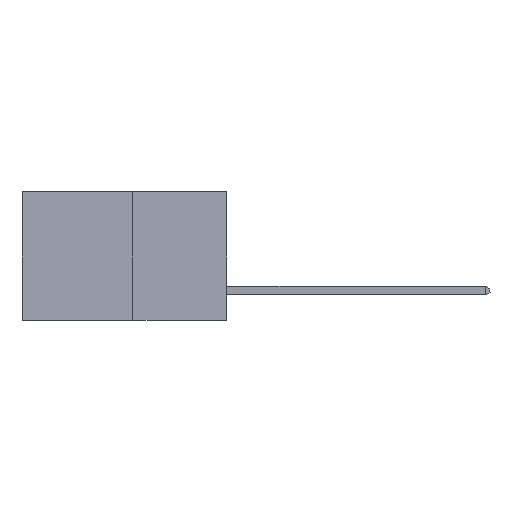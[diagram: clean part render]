
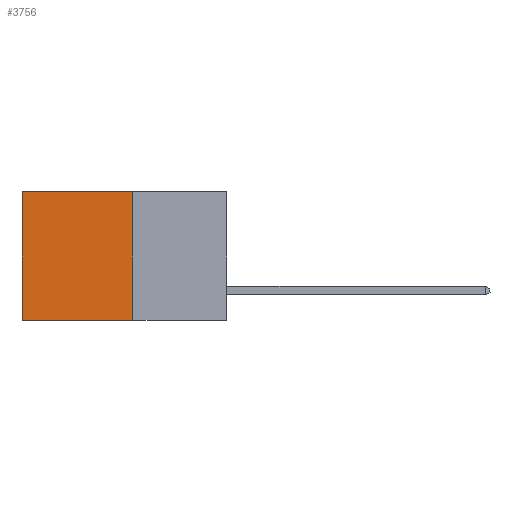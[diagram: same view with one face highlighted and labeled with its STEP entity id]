
A CAD part, left-side view. The second image highlights one B-rep face of the part: STEP entity #3756.
In plain terms, the highlighted planar face has unit normal (-1, 0, 0).
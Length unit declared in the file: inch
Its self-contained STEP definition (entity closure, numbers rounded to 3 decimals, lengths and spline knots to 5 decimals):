
#279 = VECTOR ( 'NONE', #6995, 39.37008 ) ;
#903 = VECTOR ( 'NONE', #10821, 39.37008 ) ;
#1159 = EDGE_LOOP ( 'NONE', ( #3875, #5077, #8841, #7948 ) ) ;
#1236 = VERTEX_POINT ( 'NONE', #6730 ) ;
#1949 = DIRECTION ( 'NONE',  ( 0., 0., -1. ) ) ;
#2069 = CARTESIAN_POINT ( 'NONE',  ( 0.277, 0.27, -0.37 ) ) ;
#2917 = VERTEX_POINT ( 'NONE', #6282 ) ;
#2950 = VECTOR ( 'NONE', #1949, 39.37008 ) ;
#3147 = VECTOR ( 'NONE', #10417, 39.37008 ) ;
#3756 = ADVANCED_FACE ( 'NONE', ( #9058 ), #8468, .F. ) ;
#3875 = ORIENTED_EDGE ( 'NONE', *, *, #9481, .T. ) ;
#3939 = EDGE_CURVE ( 'NONE', #10546, #2917, #5528, .T. ) ;
#4359 = AXIS2_PLACEMENT_3D ( 'NONE', #8403, #8313, #8305 ) ;
#4400 = EDGE_CURVE ( 'NONE', #1236, #10546, #7510, .T. ) ;
#4759 = VERTEX_POINT ( 'NONE', #7749 ) ;
#5077 = ORIENTED_EDGE ( 'NONE', *, *, #3939, .F. ) ;
#5528 = LINE ( 'NONE', #6834, #279 ) ;
#6083 = LINE ( 'NONE', #10022, #903 ) ;
#6282 = CARTESIAN_POINT ( 'NONE',  ( 0.277, 0.59, -0.37 ) ) ;
#6730 = CARTESIAN_POINT ( 'NONE',  ( 0.277, 0.27, 0. ) ) ;
#6834 = CARTESIAN_POINT ( 'NONE',  ( 0.277, 0.27, -0.37 ) ) ;
#6995 = DIRECTION ( 'NONE',  ( 0., 1., 0. ) ) ;
#7244 = CARTESIAN_POINT ( 'NONE',  ( 0.277, 0.27, 0. ) ) ;
#7380 = EDGE_CURVE ( 'NONE', #1236, #4759, #9361, .T. ) ;
#7510 = LINE ( 'NONE', #2069, #2950 ) ;
#7749 = CARTESIAN_POINT ( 'NONE',  ( 0.277, 0.59, 0. ) ) ;
#7948 = ORIENTED_EDGE ( 'NONE', *, *, #7380, .T. ) ;
#8305 = DIRECTION ( 'NONE',  ( 0., 0., -1. ) ) ;
#8313 = DIRECTION ( 'NONE',  ( 1., 0., 0. ) ) ;
#8403 = CARTESIAN_POINT ( 'NONE',  ( 0.277, 0.27, -0.37 ) ) ;
#8468 = PLANE ( 'NONE',  #4359 ) ;
#8841 = ORIENTED_EDGE ( 'NONE', *, *, #4400, .F. ) ;
#9058 = FACE_OUTER_BOUND ( 'NONE', #1159, .T. ) ;
#9298 = CARTESIAN_POINT ( 'NONE',  ( 0.277, 0.27, -0.37 ) ) ;
#9361 = LINE ( 'NONE', #7244, #3147 ) ;
#9481 = EDGE_CURVE ( 'NONE', #4759, #2917, #6083, .T. ) ;
#10022 = CARTESIAN_POINT ( 'NONE',  ( 0.277, 0.59, -0.37 ) ) ;
#10417 = DIRECTION ( 'NONE',  ( 0., 1., 0. ) ) ;
#10546 = VERTEX_POINT ( 'NONE', #9298 ) ;
#10821 = DIRECTION ( 'NONE',  ( 0., 0., -1. ) ) ;
